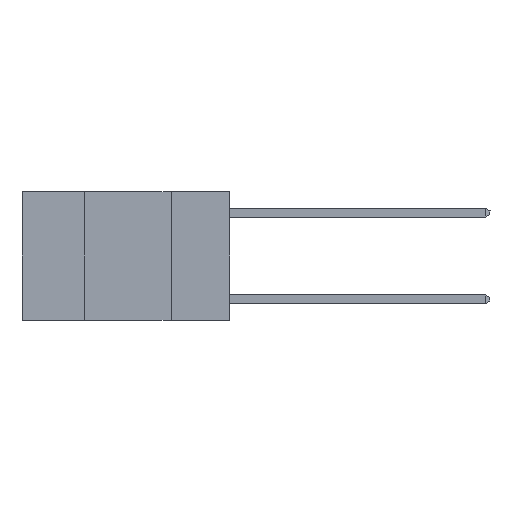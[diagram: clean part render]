
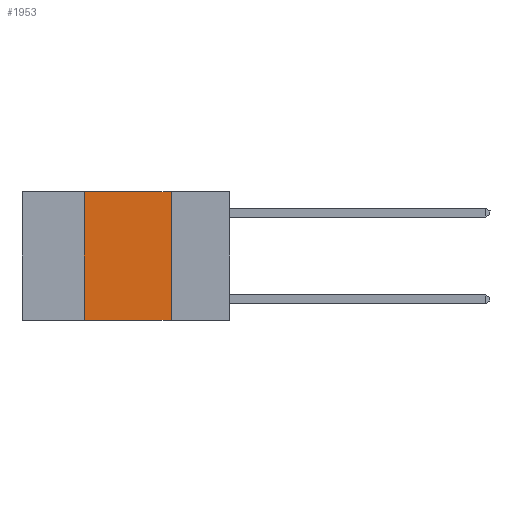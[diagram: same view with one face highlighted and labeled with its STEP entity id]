
A CAD part, left-side view. The second image highlights one B-rep face of the part: STEP entity #1953.
In plain terms, the highlighted planar face has unit normal (-1, 0, 0).
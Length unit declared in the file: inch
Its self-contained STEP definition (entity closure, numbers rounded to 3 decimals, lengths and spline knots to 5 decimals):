
#189 = LINE ( 'NONE', #4798, #8389 ) ;
#294 = ORIENTED_EDGE ( 'NONE', *, *, #556, .F. ) ;
#366 = DIRECTION ( 'NONE',  ( 1., 0., 0. ) ) ;
#556 = EDGE_CURVE ( 'NONE', #11006, #7006, #3879, .T. ) ;
#647 = LINE ( 'NONE', #10760, #10638 ) ;
#1272 = ORIENTED_EDGE ( 'NONE', *, *, #9752, .F. ) ;
#1586 = EDGE_LOOP ( 'NONE', ( #294, #4561, #1272, #5306 ) ) ;
#1953 = ADVANCED_FACE ( 'NONE', ( #11519 ), #6017, .F. ) ;
#2040 = DIRECTION ( 'NONE',  ( 0., 0., -1. ) ) ;
#2838 = CARTESIAN_POINT ( 'NONE',  ( 0., 0.42, 0. ) ) ;
#3340 = VECTOR ( 'NONE', #2040, 39.37008 ) ;
#3879 = LINE ( 'NONE', #10370, #3340 ) ;
#4561 = ORIENTED_EDGE ( 'NONE', *, *, #4563, .F. ) ;
#4563 = EDGE_CURVE ( 'NONE', #5647, #11006, #647, .T. ) ;
#4798 = CARTESIAN_POINT ( 'NONE',  ( 0., 0.42, 0. ) ) ;
#4953 = EDGE_CURVE ( 'NONE', #7721, #7006, #7003, .T. ) ;
#5133 = CARTESIAN_POINT ( 'NONE',  ( 0., 0.17, 0. ) ) ;
#5306 = ORIENTED_EDGE ( 'NONE', *, *, #4953, .T. ) ;
#5368 = CARTESIAN_POINT ( 'NONE',  ( 0., 0.17, -0.37 ) ) ;
#5647 = VERTEX_POINT ( 'NONE', #2838 ) ;
#5905 = DIRECTION ( 'NONE',  ( 0., 0., -1. ) ) ;
#6017 = PLANE ( 'NONE',  #9489 ) ;
#6160 = CARTESIAN_POINT ( 'NONE',  ( 0., 0.42, -0.37 ) ) ;
#6629 = DIRECTION ( 'NONE',  ( 0., 0., 1. ) ) ;
#7003 = LINE ( 'NONE', #11491, #9676 ) ;
#7006 = VERTEX_POINT ( 'NONE', #5368 ) ;
#7721 = VERTEX_POINT ( 'NONE', #6160 ) ;
#7908 = DIRECTION ( 'NONE',  ( 0., -1., 0. ) ) ;
#8016 = DIRECTION ( 'NONE',  ( 0., -1., 0. ) ) ;
#8389 = VECTOR ( 'NONE', #6629, 39.37008 ) ;
#9489 = AXIS2_PLACEMENT_3D ( 'NONE', #11455, #366, #5905 ) ;
#9676 = VECTOR ( 'NONE', #8016, 39.37008 ) ;
#9752 = EDGE_CURVE ( 'NONE', #7721, #5647, #189, .T. ) ;
#10370 = CARTESIAN_POINT ( 'NONE',  ( 0., 0.17, 0. ) ) ;
#10638 = VECTOR ( 'NONE', #7908, 39.37008 ) ;
#10760 = CARTESIAN_POINT ( 'NONE',  ( 0., 0.6, 0. ) ) ;
#11006 = VERTEX_POINT ( 'NONE', #5133 ) ;
#11455 = CARTESIAN_POINT ( 'NONE',  ( 0., 0.6, 0. ) ) ;
#11491 = CARTESIAN_POINT ( 'NONE',  ( 0., 0.6, -0.37 ) ) ;
#11519 = FACE_OUTER_BOUND ( 'NONE', #1586, .T. ) ;
